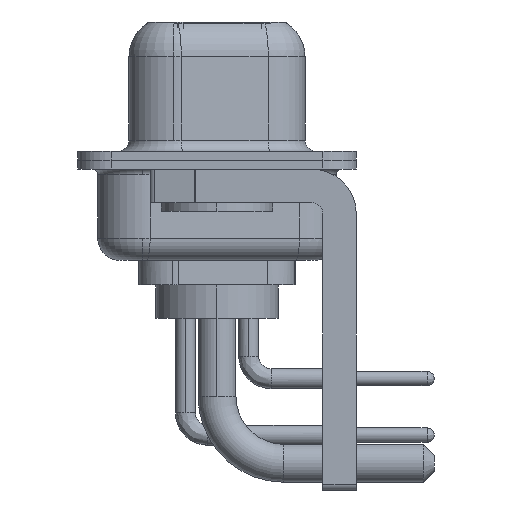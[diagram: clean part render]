
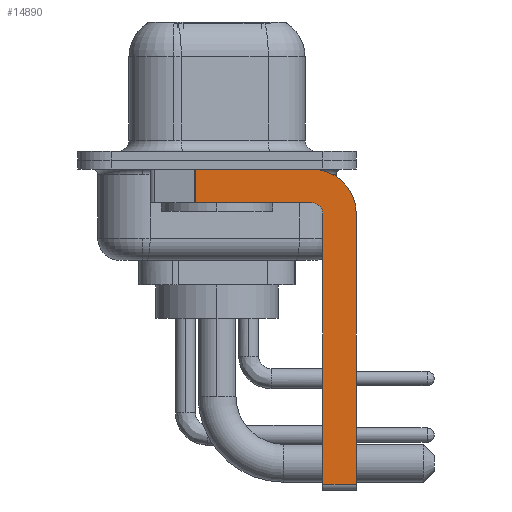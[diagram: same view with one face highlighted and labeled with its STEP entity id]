
A CAD part, left-side view. The second image highlights one B-rep face of the part: STEP entity #14890.
In plain terms, the highlighted planar face has unit normal (-1, 0, 0).
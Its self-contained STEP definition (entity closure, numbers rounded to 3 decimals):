
#384 = CARTESIAN_POINT ( 'NONE',  ( -2.9, 0.978, -1.9 ) ) ;
#467 = CARTESIAN_POINT ( 'NONE',  ( -2.9, -4.75, -2.4 ) ) ;
#987 = VECTOR ( 'NONE', #7212, 1000. ) ;
#1095 = CIRCLE ( 'NONE', #3467, 0.5 ) ;
#1245 = CARTESIAN_POINT ( 'NONE',  ( -2.9, -4.25, -2.4 ) ) ;
#1256 = EDGE_CURVE ( 'NONE', #7851, #2742, #11985, .T. ) ;
#1534 = VERTEX_POINT ( 'NONE', #20875 ) ;
#1750 = CARTESIAN_POINT ( 'NONE',  ( -2.9, -4.75, -14.55 ) ) ;
#1795 = DIRECTION ( 'NONE',  ( 0., 0., -1. ) ) ;
#2104 = DIRECTION ( 'NONE',  ( 1., 0., 0. ) ) ;
#2742 = VERTEX_POINT ( 'NONE', #467 ) ;
#2947 = DIRECTION ( 'NONE',  ( -1., 0., 0. ) ) ;
#3467 = AXIS2_PLACEMENT_3D ( 'NONE', #20467, #2947, #19086 ) ;
#4007 = EDGE_CURVE ( 'NONE', #8376, #13539, #15116, .T. ) ;
#4029 = LINE ( 'NONE', #10707, #4397 ) ;
#4397 = VECTOR ( 'NONE', #9012, 1000. ) ;
#4553 = CARTESIAN_POINT ( 'NONE',  ( -2.9, -4.25, -1.9 ) ) ;
#4645 = DIRECTION ( 'NONE',  ( 0., -1., 0. ) ) ;
#4925 = EDGE_CURVE ( 'NONE', #20121, #1534, #4029, .T. ) ;
#4974 = FACE_OUTER_BOUND ( 'NONE', #15111, .T. ) ;
#5012 = ORIENTED_EDGE ( 'NONE', *, *, #7795, .T. ) ;
#5122 = AXIS2_PLACEMENT_3D ( 'NONE', #1245, #14194, #20778 ) ;
#5188 = EDGE_CURVE ( 'NONE', #9170, #8367, #14196, .T. ) ;
#5319 = CARTESIAN_POINT ( 'NONE',  ( -2.9, -6.25, -2.4 ) ) ;
#5345 = ORIENTED_EDGE ( 'NONE', *, *, #20759, .F. ) ;
#5448 = DIRECTION ( 'NONE',  ( 0., 1., 0. ) ) ;
#5859 = VECTOR ( 'NONE', #5448, 1000. ) ;
#5888 = ORIENTED_EDGE ( 'NONE', *, *, #6618, .T. ) ;
#6618 = EDGE_CURVE ( 'NONE', #9170, #13539, #14093, .T. ) ;
#6873 = EDGE_CURVE ( 'NONE', #8367, #20121, #16652, .T. ) ;
#7212 = DIRECTION ( 'NONE',  ( 0., 0., 1. ) ) ;
#7795 = EDGE_CURVE ( 'NONE', #7851, #1534, #11929, .T. ) ;
#7851 = VERTEX_POINT ( 'NONE', #1750 ) ;
#8367 = VERTEX_POINT ( 'NONE', #19867 ) ;
#8376 = VERTEX_POINT ( 'NONE', #4553 ) ;
#8445 = CARTESIAN_POINT ( 'NONE',  ( -2.9, 0.978, -0.4 ) ) ;
#8600 = CARTESIAN_POINT ( 'NONE',  ( -2.9, -4.75, -14.8 ) ) ;
#9012 = DIRECTION ( 'NONE',  ( 0., 0., -1. ) ) ;
#9170 = VERTEX_POINT ( 'NONE', #8445 ) ;
#9553 = VECTOR ( 'NONE', #14802, 1000. ) ;
#9854 = PLANE ( 'NONE',  #13209 ) ;
#10705 = DIRECTION ( 'NONE',  ( 0., 0., -1. ) ) ;
#10707 = CARTESIAN_POINT ( 'NONE',  ( -2.9, -6.25, -2.4 ) ) ;
#11929 = LINE ( 'NONE', #19582, #9553 ) ;
#11985 = LINE ( 'NONE', #8600, #987 ) ;
#12861 = ORIENTED_EDGE ( 'NONE', *, *, #5188, .F. ) ;
#13209 = AXIS2_PLACEMENT_3D ( 'NONE', #16339, #2104, #1795 ) ;
#13539 = VERTEX_POINT ( 'NONE', #384 ) ;
#14093 = LINE ( 'NONE', #17185, #17180 ) ;
#14194 = DIRECTION ( 'NONE',  ( 1., 0., 0. ) ) ;
#14196 = LINE ( 'NONE', #20669, #16567 ) ;
#14802 = DIRECTION ( 'NONE',  ( 0., -1., 0. ) ) ;
#14890 = ADVANCED_FACE ( 'NONE', ( #4974 ), #9854, .F. ) ;
#15111 = EDGE_LOOP ( 'NONE', ( #12861, #5888, #15775, #5345, #18705, #5012, #18448, #15885 ) ) ;
#15116 = LINE ( 'NONE', #19983, #5859 ) ;
#15775 = ORIENTED_EDGE ( 'NONE', *, *, #4007, .F. ) ;
#15885 = ORIENTED_EDGE ( 'NONE', *, *, #6873, .F. ) ;
#16339 = CARTESIAN_POINT ( 'NONE',  ( -2.9, -4.25, -2.4 ) ) ;
#16567 = VECTOR ( 'NONE', #4645, 1000. ) ;
#16652 = CIRCLE ( 'NONE', #5122, 2. ) ;
#17180 = VECTOR ( 'NONE', #10705, 1000. ) ;
#17185 = CARTESIAN_POINT ( 'NONE',  ( -2.9, 0.978, -1.9 ) ) ;
#18448 = ORIENTED_EDGE ( 'NONE', *, *, #4925, .F. ) ;
#18705 = ORIENTED_EDGE ( 'NONE', *, *, #1256, .F. ) ;
#19086 = DIRECTION ( 'NONE',  ( 0., 0., 1. ) ) ;
#19582 = CARTESIAN_POINT ( 'NONE',  ( -2.9, -4.25, -14.55 ) ) ;
#19867 = CARTESIAN_POINT ( 'NONE',  ( -2.9, -4.25, -0.4 ) ) ;
#19983 = CARTESIAN_POINT ( 'NONE',  ( -2.9, -4.25, -1.9 ) ) ;
#20121 = VERTEX_POINT ( 'NONE', #5319 ) ;
#20467 = CARTESIAN_POINT ( 'NONE',  ( -2.9, -4.25, -2.4 ) ) ;
#20669 = CARTESIAN_POINT ( 'NONE',  ( -2.9, 3., -0.4 ) ) ;
#20759 = EDGE_CURVE ( 'NONE', #2742, #8376, #1095, .T. ) ;
#20778 = DIRECTION ( 'NONE',  ( 0., 0., -1. ) ) ;
#20875 = CARTESIAN_POINT ( 'NONE',  ( -2.9, -6.25, -14.55 ) ) ;
